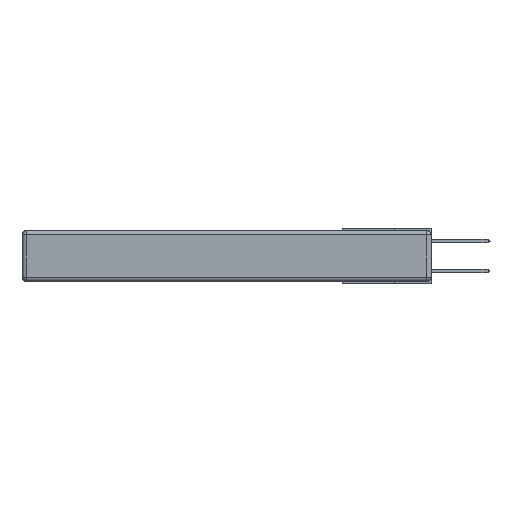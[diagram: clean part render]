
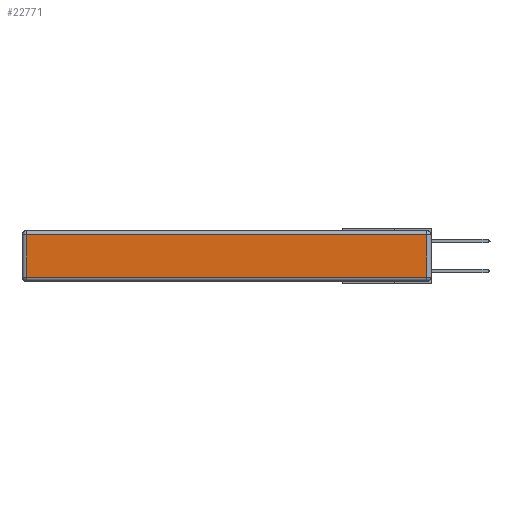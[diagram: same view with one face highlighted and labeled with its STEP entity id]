
A CAD part, left-side view. The second image highlights one B-rep face of the part: STEP entity #22771.
In plain terms, the highlighted planar face has unit normal (-1, 0, 0).
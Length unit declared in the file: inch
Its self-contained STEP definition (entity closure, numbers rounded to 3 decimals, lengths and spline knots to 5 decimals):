
#1062 = PLANE ( 'NONE',  #3016 ) ;
#3016 = AXIS2_PLACEMENT_3D ( 'NONE', #15900, #15991, #18030 ) ;
#4175 = ORIENTED_EDGE ( 'NONE', *, *, #13064, .T. ) ;
#5826 = CARTESIAN_POINT ( 'NONE',  ( 0., 2.72, -0.313 ) ) ;
#5849 = VECTOR ( 'NONE', #20546, 39.37008 ) ;
#6339 = VERTEX_POINT ( 'NONE', #5826 ) ;
#7198 = LINE ( 'NONE', #26922, #5849 ) ;
#9716 = EDGE_CURVE ( 'NONE', #14808, #20375, #15404, .T. ) ;
#10304 = CARTESIAN_POINT ( 'NONE',  ( 0., 2.75, -0.03 ) ) ;
#10867 = ORIENTED_EDGE ( 'NONE', *, *, #17555, .T. ) ;
#10888 = EDGE_LOOP ( 'NONE', ( #4175, #20469, #12367, #10867 ) ) ;
#11372 = VECTOR ( 'NONE', #13708, 39.37008 ) ;
#11403 = VECTOR ( 'NONE', #16880, 39.37008 ) ;
#11885 = DIRECTION ( 'NONE',  ( 0., -1., 0. ) ) ;
#12152 = CARTESIAN_POINT ( 'NONE',  ( 0., 0., -0.313 ) ) ;
#12367 = ORIENTED_EDGE ( 'NONE', *, *, #9716, .T. ) ;
#12754 = LINE ( 'NONE', #12152, #16033 ) ;
#13064 = EDGE_CURVE ( 'NONE', #6339, #16762, #12754, .T. ) ;
#13688 = EDGE_CURVE ( 'NONE', #16762, #14808, #25375, .T. ) ;
#13708 = DIRECTION ( 'NONE',  ( 0., 0., 1. ) ) ;
#14808 = VERTEX_POINT ( 'NONE', #26423 ) ;
#15404 = LINE ( 'NONE', #10304, #11403 ) ;
#15900 = CARTESIAN_POINT ( 'NONE',  ( 0., 0., -0.343 ) ) ;
#15991 = DIRECTION ( 'NONE',  ( -1., 0., 0. ) ) ;
#16033 = VECTOR ( 'NONE', #11885, 39.37008 ) ;
#16762 = VERTEX_POINT ( 'NONE', #19506 ) ;
#16880 = DIRECTION ( 'NONE',  ( 0., 1., 0. ) ) ;
#17555 = EDGE_CURVE ( 'NONE', #20375, #6339, #7198, .T. ) ;
#18030 = DIRECTION ( 'NONE',  ( 0., 0., 1. ) ) ;
#19506 = CARTESIAN_POINT ( 'NONE',  ( 0., 0.03, -0.313 ) ) ;
#20375 = VERTEX_POINT ( 'NONE', #27095 ) ;
#20469 = ORIENTED_EDGE ( 'NONE', *, *, #13688, .T. ) ;
#20546 = DIRECTION ( 'NONE',  ( 0., 0., -1. ) ) ;
#22771 = ADVANCED_FACE ( 'NONE', ( #26562 ), #1062, .T. ) ;
#24605 = CARTESIAN_POINT ( 'NONE',  ( 0., 0.03, -0.343 ) ) ;
#25375 = LINE ( 'NONE', #24605, #11372 ) ;
#26423 = CARTESIAN_POINT ( 'NONE',  ( 0., 0.03, -0.03 ) ) ;
#26562 = FACE_OUTER_BOUND ( 'NONE', #10888, .T. ) ;
#26922 = CARTESIAN_POINT ( 'NONE',  ( 0., 2.72, -0.343 ) ) ;
#27095 = CARTESIAN_POINT ( 'NONE',  ( 0., 2.72, -0.03 ) ) ;
